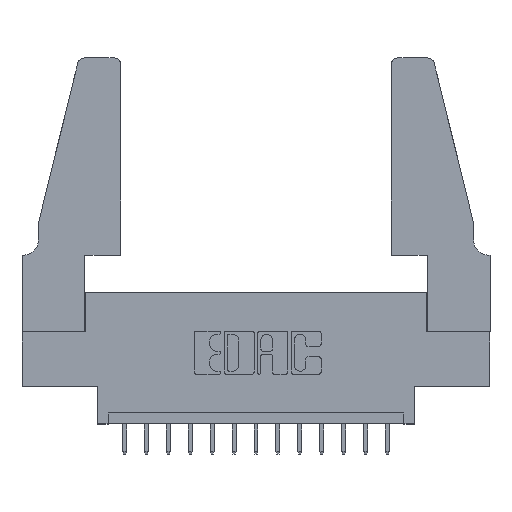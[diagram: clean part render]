
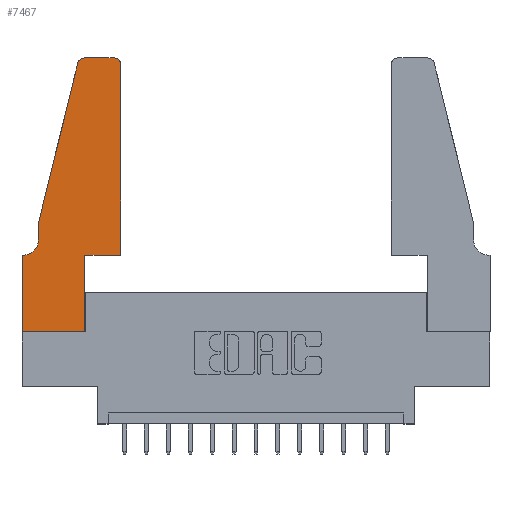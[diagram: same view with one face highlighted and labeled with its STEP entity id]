
A CAD part, top view. The second image highlights one B-rep face of the part: STEP entity #7467.
In plain terms, the highlighted planar face has unit normal (0, 0, 1).
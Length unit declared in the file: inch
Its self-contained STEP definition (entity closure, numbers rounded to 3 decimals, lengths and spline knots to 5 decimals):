
#536 = CARTESIAN_POINT ( 'NONE',  ( 0., 0., 0.37 ) ) ;
#802 = CARTESIAN_POINT ( 'NONE',  ( 0.284, 1.22, 0.37 ) ) ;
#878 = CARTESIAN_POINT ( 'NONE',  ( 0.2865, 0.35, 0.37 ) ) ;
#970 = EDGE_CURVE ( 'NONE', #5464, #7548, #7551, .T. ) ;
#1128 = DIRECTION ( 'NONE',  ( 0., -1., 0. ) ) ;
#1199 = EDGE_CURVE ( 'NONE', #14935, #9325, #15696, .T. ) ;
#1491 = LINE ( 'NONE', #6300, #10035 ) ;
#1639 = LINE ( 'NONE', #4078, #10733 ) ;
#1850 = DIRECTION ( 'NONE',  ( 0., 1., 0. ) ) ;
#1872 = DIRECTION ( 'NONE',  ( 0., -1., 0. ) ) ;
#2213 = CARTESIAN_POINT ( 'NONE',  ( 0.0755, 0.35, 0.37 ) ) ;
#2243 = CIRCLE ( 'NONE', #15510, 0.03 ) ;
#2350 = LINE ( 'NONE', #5834, #10267 ) ;
#2685 = EDGE_CURVE ( 'NONE', #8003, #9198, #9556, .T. ) ;
#2915 = ORIENTED_EDGE ( 'NONE', *, *, #10119, .T. ) ;
#3069 = DIRECTION ( 'NONE',  ( 1., 0., 0. ) ) ;
#3192 = EDGE_CURVE ( 'NONE', #7548, #4729, #8316, .T. ) ;
#3480 = EDGE_CURVE ( 'NONE', #4729, #13141, #1639, .T. ) ;
#4078 = CARTESIAN_POINT ( 'NONE',  ( 0., 0., 0.37 ) ) ;
#4365 = CARTESIAN_POINT ( 'NONE',  ( 0.4205, 1.25, 0.37 ) ) ;
#4729 = VERTEX_POINT ( 'NONE', #12875 ) ;
#4958 = EDGE_LOOP ( 'NONE', ( #7462, #2915, #8252, #13811, #6014, #10217, #5492, #6149, #10396, #15872, #5338, #14454 ) ) ;
#4967 = EDGE_CURVE ( 'NONE', #12092, #9724, #9691, .T. ) ;
#4999 = VECTOR ( 'NONE', #5872, 39.37008 ) ;
#5329 = AXIS2_PLACEMENT_3D ( 'NONE', #13639, #12723, #13717 ) ;
#5338 = ORIENTED_EDGE ( 'NONE', *, *, #4967, .T. ) ;
#5464 = VERTEX_POINT ( 'NONE', #12326 ) ;
#5475 = CARTESIAN_POINT ( 'NONE',  ( 0.4505, 0.35, 0.37 ) ) ;
#5492 = ORIENTED_EDGE ( 'NONE', *, *, #3480, .T. ) ;
#5717 = AXIS2_PLACEMENT_3D ( 'NONE', #10154, #9914, #11375 ) ;
#5746 = DIRECTION ( 'NONE',  ( 1., 0., 0. ) ) ;
#5834 = CARTESIAN_POINT ( 'NONE',  ( 0.0755, 0.5, 0.37 ) ) ;
#5872 = DIRECTION ( 'NONE',  ( -1., 0., 0. ) ) ;
#5968 = VECTOR ( 'NONE', #9855, 39.37008 ) ;
#6014 = ORIENTED_EDGE ( 'NONE', *, *, #970, .T. ) ;
#6149 = ORIENTED_EDGE ( 'NONE', *, *, #16030, .T. ) ;
#6220 = EDGE_CURVE ( 'NONE', #10101, #14782, #12051, .T. ) ;
#6300 = CARTESIAN_POINT ( 'NONE',  ( 0.4505, 0.35, 0.37 ) ) ;
#7327 = EDGE_CURVE ( 'NONE', #9325, #5464, #2350, .T. ) ;
#7462 = ORIENTED_EDGE ( 'NONE', *, *, #6220, .T. ) ;
#7467 = ADVANCED_FACE ( 'NONE', ( #14207 ), #12903, .T. ) ;
#7548 = VERTEX_POINT ( 'NONE', #10553 ) ;
#7551 = CIRCLE ( 'NONE', #5717, 0.07 ) ;
#7959 = CARTESIAN_POINT ( 'NONE',  ( 0., 0.35, 0.37 ) ) ;
#8003 = VERTEX_POINT ( 'NONE', #10834 ) ;
#8252 = ORIENTED_EDGE ( 'NONE', *, *, #1199, .T. ) ;
#8316 = LINE ( 'NONE', #2213, #14608 ) ;
#8461 = CIRCLE ( 'NONE', #5329, 0.03 ) ;
#9102 = EDGE_CURVE ( 'NONE', #9724, #10101, #8461, .T. ) ;
#9149 = CARTESIAN_POINT ( 'NONE',  ( 0.0755, 0.5, 0.37 ) ) ;
#9198 = VERTEX_POINT ( 'NONE', #14941 ) ;
#9325 = VERTEX_POINT ( 'NONE', #9149 ) ;
#9327 = DIRECTION ( 'NONE',  ( 0., 0., 1. ) ) ;
#9428 = CARTESIAN_POINT ( 'NONE',  ( 0., 0., 0.37 ) ) ;
#9478 = CARTESIAN_POINT ( 'NONE',  ( 0.0755, 0.5, 0.37 ) ) ;
#9556 = LINE ( 'NONE', #878, #15661 ) ;
#9589 = EDGE_CURVE ( 'NONE', #9198, #12092, #1491, .T. ) ;
#9668 = DIRECTION ( 'NONE',  ( 1., 0., 0. ) ) ;
#9691 = LINE ( 'NONE', #12362, #5968 ) ;
#9721 = DIRECTION ( 'NONE',  ( -0.239, -0.971, 0. ) ) ;
#9724 = VERTEX_POINT ( 'NONE', #14338 ) ;
#9744 = CARTESIAN_POINT ( 'NONE',  ( 0.25487, 1.22718, 0.37 ) ) ;
#9855 = DIRECTION ( 'NONE',  ( 0., 1., 0. ) ) ;
#9914 = DIRECTION ( 'NONE',  ( 0., 0., -1. ) ) ;
#10035 = VECTOR ( 'NONE', #11257, 39.37008 ) ;
#10101 = VERTEX_POINT ( 'NONE', #4365 ) ;
#10119 = EDGE_CURVE ( 'NONE', #14782, #14935, #2243, .T. ) ;
#10154 = CARTESIAN_POINT ( 'NONE',  ( 0.0055, 0.42, 0.37 ) ) ;
#10217 = ORIENTED_EDGE ( 'NONE', *, *, #3192, .T. ) ;
#10251 = CARTESIAN_POINT ( 'NONE',  ( 0.284, 1.25, 0.37 ) ) ;
#10267 = VECTOR ( 'NONE', #1128, 39.37008 ) ;
#10396 = ORIENTED_EDGE ( 'NONE', *, *, #2685, .T. ) ;
#10553 = CARTESIAN_POINT ( 'NONE',  ( 0.0055, 0.35, 0.37 ) ) ;
#10733 = VECTOR ( 'NONE', #1872, 39.37008 ) ;
#10834 = CARTESIAN_POINT ( 'NONE',  ( 0.2865, 0., 0.37 ) ) ;
#10928 = VECTOR ( 'NONE', #9721, 39.37008 ) ;
#11257 = DIRECTION ( 'NONE',  ( 1., 0., 0. ) ) ;
#11375 = DIRECTION ( 'NONE',  ( -1., 0., 0. ) ) ;
#11544 = AXIS2_PLACEMENT_3D ( 'NONE', #7959, #15610, #3069 ) ;
#12030 = LINE ( 'NONE', #9428, #14827 ) ;
#12051 = LINE ( 'NONE', #13048, #4999 ) ;
#12092 = VERTEX_POINT ( 'NONE', #5475 ) ;
#12205 = DIRECTION ( 'NONE',  ( -1., 0., 0. ) ) ;
#12326 = CARTESIAN_POINT ( 'NONE',  ( 0.0755, 0.42, 0.37 ) ) ;
#12362 = CARTESIAN_POINT ( 'NONE',  ( 0.4505, 0.35, 0.37 ) ) ;
#12723 = DIRECTION ( 'NONE',  ( 0., 0., 1. ) ) ;
#12875 = CARTESIAN_POINT ( 'NONE',  ( 0., 0.35, 0.37 ) ) ;
#12903 = PLANE ( 'NONE',  #11544 ) ;
#13048 = CARTESIAN_POINT ( 'NONE',  ( 0.2605, 1.25, 0.37 ) ) ;
#13141 = VERTEX_POINT ( 'NONE', #536 ) ;
#13639 = CARTESIAN_POINT ( 'NONE',  ( 0.4205, 1.22, 0.37 ) ) ;
#13717 = DIRECTION ( 'NONE',  ( 1., 0., 0. ) ) ;
#13811 = ORIENTED_EDGE ( 'NONE', *, *, #7327, .T. ) ;
#14207 = FACE_OUTER_BOUND ( 'NONE', #4958, .T. ) ;
#14338 = CARTESIAN_POINT ( 'NONE',  ( 0.4505, 1.22, 0.37 ) ) ;
#14454 = ORIENTED_EDGE ( 'NONE', *, *, #9102, .T. ) ;
#14608 = VECTOR ( 'NONE', #12205, 39.37008 ) ;
#14782 = VERTEX_POINT ( 'NONE', #10251 ) ;
#14827 = VECTOR ( 'NONE', #9668, 39.37008 ) ;
#14935 = VERTEX_POINT ( 'NONE', #9744 ) ;
#14941 = CARTESIAN_POINT ( 'NONE',  ( 0.2865, 0.35, 0.37 ) ) ;
#15510 = AXIS2_PLACEMENT_3D ( 'NONE', #802, #9327, #5746 ) ;
#15610 = DIRECTION ( 'NONE',  ( 0., 0., 1. ) ) ;
#15661 = VECTOR ( 'NONE', #1850, 39.37008 ) ;
#15696 = LINE ( 'NONE', #9478, #10928 ) ;
#15872 = ORIENTED_EDGE ( 'NONE', *, *, #9589, .T. ) ;
#16030 = EDGE_CURVE ( 'NONE', #13141, #8003, #12030, .T. ) ;
